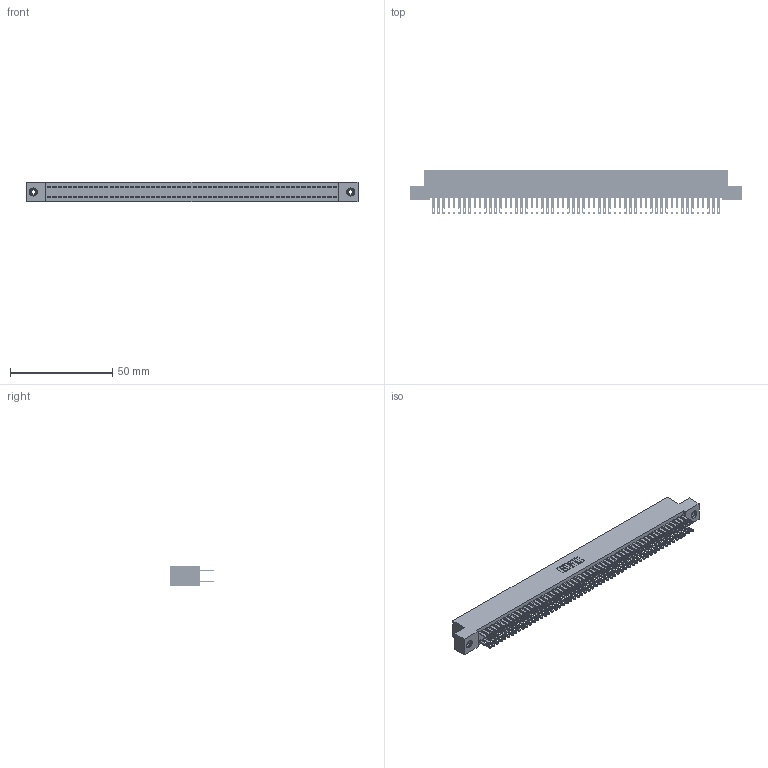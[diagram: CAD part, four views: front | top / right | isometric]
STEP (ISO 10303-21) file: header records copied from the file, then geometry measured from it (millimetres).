
FILE_DESCRIPTION (( 'STEP AP203' ), '1' );
FILE_NAME ('892-112-500-208.STEP', '2020-09-21T22:03:02', ( '' ), ( '' ), 'SwSTEP 2.0', 'SolidWorks 2020', '' );
FILE_SCHEMA (( 'CONFIG_CONTROL_DESIGN' ));
Length unit declared in the file: inch
Products named in the file (4): 842 Part_TI; 892-112-500-208; 345-292-001_345-293-100; 345-250-001_345-250-003-102
Assembly tree (115 placements, depth 2):
  892-112-500-208
    842 Part_TI
    345-292-001_345-293-100  x112
    345-250-001_345-250-003-102  x2
Bounding box: 162.56 x 21.85 x 9.4 mm (x, y, z)
Volume: 15008.8 mm3; surface area: 25858.2 mm2
Topology: 115 solids, 115 shells, 5546 faces, 16899 edges, 11258 vertices
Faces by surface type: plane 3458, cylinder 2072, cone 12, torus 4
Entity records: 35200 total; most frequent: CARTESIAN_POINT 5797, ORIENTED_EDGE 5726, DIRECTION 4961, EDGE_CURVE 2863, VECTOR 2711, LINE 2711, VERTEX_POINT 1904, AXIS2_PLACEMENT_3D 1125
